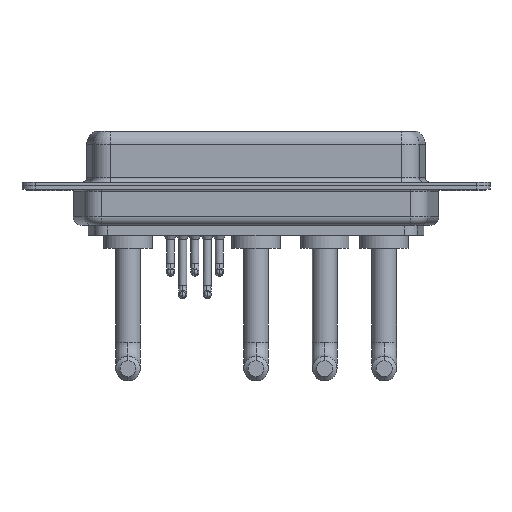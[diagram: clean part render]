
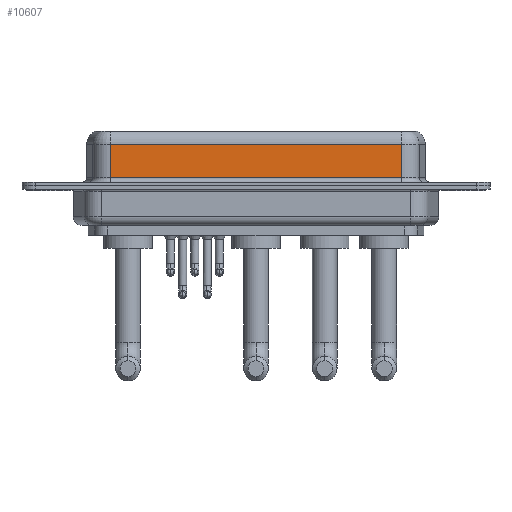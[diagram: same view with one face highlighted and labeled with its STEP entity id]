
A CAD part, front view. The second image highlights one B-rep face of the part: STEP entity #10607.
In plain terms, the highlighted planar face has unit normal (0, -1, 0).
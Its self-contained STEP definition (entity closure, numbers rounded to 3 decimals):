
#229 = DIRECTION ( 'NONE',  ( 0., 0., -1. ) ) ;
#574 = VECTOR ( 'NONE', #229, 1000. ) ;
#1167 = LINE ( 'NONE', #10959, #574 ) ;
#1168 = CARTESIAN_POINT ( 'NONE',  ( 40.037, -3.95, 4.65 ) ) ;
#1474 = FACE_OUTER_BOUND ( 'NONE', #9488, .T. ) ;
#1552 = PLANE ( 'NONE',  #6279 ) ;
#1839 = DIRECTION ( 'NONE',  ( 0., 0., 1. ) ) ;
#2444 = CARTESIAN_POINT ( 'NONE',  ( 7.013, -3.95, 0.9 ) ) ;
#3130 = CARTESIAN_POINT ( 'NONE',  ( 7.013, -3.95, 6.4 ) ) ;
#4061 = ORIENTED_EDGE ( 'NONE', *, *, #6981, .T. ) ;
#4459 = VECTOR ( 'NONE', #9228, 1000. ) ;
#5143 = DIRECTION ( 'NONE',  ( 0., 1., 0. ) ) ;
#5856 = VECTOR ( 'NONE', #9784, 1000. ) ;
#6180 = CARTESIAN_POINT ( 'NONE',  ( 40.037, -3.95, 4.65 ) ) ;
#6279 = AXIS2_PLACEMENT_3D ( 'NONE', #13509, #5143, #1839 ) ;
#6911 = CARTESIAN_POINT ( 'NONE',  ( 40.037, -3.95, 0.9 ) ) ;
#6981 = EDGE_CURVE ( 'NONE', #13349, #15235, #12527, .T. ) ;
#6984 = VERTEX_POINT ( 'NONE', #10333 ) ;
#7121 = VERTEX_POINT ( 'NONE', #1168 ) ;
#7365 = LINE ( 'NONE', #6180, #5856 ) ;
#9228 = DIRECTION ( 'NONE',  ( 0., 0., -1. ) ) ;
#9255 = ORIENTED_EDGE ( 'NONE', *, *, #11146, .T. ) ;
#9488 = EDGE_LOOP ( 'NONE', ( #9567, #13784, #4061, #9255 ) ) ;
#9567 = ORIENTED_EDGE ( 'NONE', *, *, #13007, .F. ) ;
#9784 = DIRECTION ( 'NONE',  ( -1., 0., 0. ) ) ;
#10333 = CARTESIAN_POINT ( 'NONE',  ( 40.037, -3.95, 0.9 ) ) ;
#10607 = ADVANCED_FACE ( 'NONE', ( #1474 ), #1552, .F. ) ;
#10959 = CARTESIAN_POINT ( 'NONE',  ( 40.037, -3.95, 6.4 ) ) ;
#11146 = EDGE_CURVE ( 'NONE', #15235, #6984, #13945, .T. ) ;
#12527 = LINE ( 'NONE', #3130, #4459 ) ;
#13007 = EDGE_CURVE ( 'NONE', #7121, #6984, #1167, .T. ) ;
#13266 = CARTESIAN_POINT ( 'NONE',  ( 7.013, -3.95, 4.65 ) ) ;
#13349 = VERTEX_POINT ( 'NONE', #13266 ) ;
#13498 = VECTOR ( 'NONE', #15268, 1000. ) ;
#13509 = CARTESIAN_POINT ( 'NONE',  ( 40.037, -3.95, 6.4 ) ) ;
#13784 = ORIENTED_EDGE ( 'NONE', *, *, #14608, .T. ) ;
#13945 = LINE ( 'NONE', #6911, #13498 ) ;
#14608 = EDGE_CURVE ( 'NONE', #7121, #13349, #7365, .T. ) ;
#15235 = VERTEX_POINT ( 'NONE', #2444 ) ;
#15268 = DIRECTION ( 'NONE',  ( 1., 0., 0. ) ) ;
